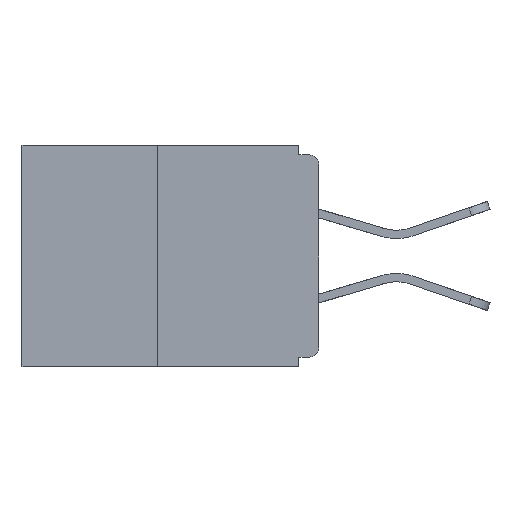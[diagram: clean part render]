
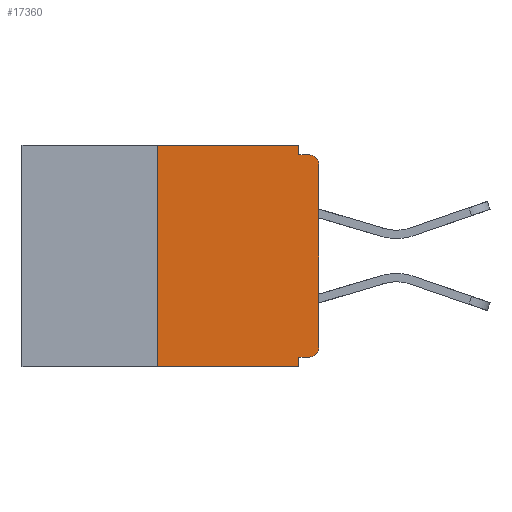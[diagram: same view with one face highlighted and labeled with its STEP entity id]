
A CAD part, left-side view. The second image highlights one B-rep face of the part: STEP entity #17360.
In plain terms, the highlighted planar face has unit normal (-1, 0, 0).
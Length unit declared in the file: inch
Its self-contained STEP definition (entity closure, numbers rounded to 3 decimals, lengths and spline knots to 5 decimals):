
#166 = ORIENTED_EDGE ( 'NONE', *, *, #1238, .T. ) ;
#215 = CARTESIAN_POINT ( 'NONE',  ( 0., 0., -0.328 ) ) ;
#246 = ORIENTED_EDGE ( 'NONE', *, *, #18057, .T. ) ;
#530 = VECTOR ( 'NONE', #8843, 39.37008 ) ;
#594 = DIRECTION ( 'NONE',  ( 0., 0., -1. ) ) ;
#1238 = EDGE_CURVE ( 'NONE', #21422, #5049, #30726, .T. ) ;
#1632 = VERTEX_POINT ( 'NONE', #28613 ) ;
#2028 = CARTESIAN_POINT ( 'NONE',  ( 0., 0., -0.313 ) ) ;
#2409 = ORIENTED_EDGE ( 'NONE', *, *, #9950, .F. ) ;
#2642 = AXIS2_PLACEMENT_3D ( 'NONE', #22882, #27794, #13150 ) ;
#2669 = CARTESIAN_POINT ( 'NONE',  ( 0., 0.015, -0.03 ) ) ;
#3594 = AXIS2_PLACEMENT_3D ( 'NONE', #27249, #15269, #594 ) ;
#4149 = VERTEX_POINT ( 'NONE', #10280 ) ;
#4864 = VERTEX_POINT ( 'NONE', #16593 ) ;
#5049 = VERTEX_POINT ( 'NONE', #30414 ) ;
#5520 = LINE ( 'NONE', #11395, #530 ) ;
#6552 = CARTESIAN_POINT ( 'NONE',  ( 0., 0.25, -0.343 ) ) ;
#7252 = EDGE_CURVE ( 'NONE', #4864, #5049, #5520, .T. ) ;
#7854 = VERTEX_POINT ( 'NONE', #2028 ) ;
#7888 = DIRECTION ( 'NONE',  ( 0., 0., -1. ) ) ;
#8566 = ORIENTED_EDGE ( 'NONE', *, *, #23306, .F. ) ;
#8618 = VECTOR ( 'NONE', #13808, 39.37008 ) ;
#8843 = DIRECTION ( 'NONE',  ( 0., 0., -1. ) ) ;
#9936 = VERTEX_POINT ( 'NONE', #29836 ) ;
#9950 = EDGE_CURVE ( 'NONE', #28685, #4864, #17190, .T. ) ;
#10280 = CARTESIAN_POINT ( 'NONE',  ( 0., 0.031, 0. ) ) ;
#10891 = DIRECTION ( 'NONE',  ( 0., -1., 0. ) ) ;
#10930 = LINE ( 'NONE', #18303, #8618 ) ;
#11076 = ORIENTED_EDGE ( 'NONE', *, *, #7252, .F. ) ;
#11395 = CARTESIAN_POINT ( 'NONE',  ( 0., 0.031, -0.343 ) ) ;
#11702 = VECTOR ( 'NONE', #31525, 39.37008 ) ;
#12018 = FACE_OUTER_BOUND ( 'NONE', #13596, .T. ) ;
#12447 = EDGE_CURVE ( 'NONE', #7854, #9936, #10930, .T. ) ;
#12721 = CARTESIAN_POINT ( 'NONE',  ( 0., 0.031, 0. ) ) ;
#13150 = DIRECTION ( 'NONE',  ( 0., 0., -1. ) ) ;
#13263 = CARTESIAN_POINT ( 'NONE',  ( 0., 0., -0.015 ) ) ;
#13403 = VECTOR ( 'NONE', #15731, 39.37008 ) ;
#13472 = EDGE_CURVE ( 'NONE', #1632, #30831, #26782, .T. ) ;
#13555 = ORIENTED_EDGE ( 'NONE', *, *, #15837, .F. ) ;
#13568 = CARTESIAN_POINT ( 'NONE',  ( 0., 0.46, 0. ) ) ;
#13596 = EDGE_LOOP ( 'NONE', ( #8566, #13555, #166, #11076, #2409, #246, #28429, #24397, #29983, #27112 ) ) ;
#13808 = DIRECTION ( 'NONE',  ( 0., 0., 1. ) ) ;
#14396 = EDGE_CURVE ( 'NONE', #9936, #30831, #28247, .T. ) ;
#14559 = CARTESIAN_POINT ( 'NONE',  ( 0., 0.25, 0. ) ) ;
#14901 = DIRECTION ( 'NONE',  ( 0., 1., 0. ) ) ;
#15269 = DIRECTION ( 'NONE',  ( -1., 0., 0. ) ) ;
#15716 = PLANE ( 'NONE',  #2642 ) ;
#15731 = DIRECTION ( 'NONE',  ( 0., -1., 0. ) ) ;
#15837 = EDGE_CURVE ( 'NONE', #21422, #19242, #24369, .T. ) ;
#16593 = CARTESIAN_POINT ( 'NONE',  ( 0., 0.031, -0.328 ) ) ;
#16851 = LINE ( 'NONE', #13568, #21045 ) ;
#17190 = LINE ( 'NONE', #215, #27528 ) ;
#17360 = ADVANCED_FACE ( 'NONE', ( #12018 ), #15716, .F. ) ;
#18057 = EDGE_CURVE ( 'NONE', #28685, #7854, #22308, .T. ) ;
#18303 = CARTESIAN_POINT ( 'NONE',  ( 0., 0., 0. ) ) ;
#19242 = VERTEX_POINT ( 'NONE', #27260 ) ;
#19511 = VECTOR ( 'NONE', #29917, 39.37008 ) ;
#21045 = VECTOR ( 'NONE', #10891, 39.37008 ) ;
#21422 = VERTEX_POINT ( 'NONE', #6552 ) ;
#22308 = CIRCLE ( 'NONE', #3594, 0.015 ) ;
#22882 = CARTESIAN_POINT ( 'NONE',  ( 0., 0.46, 0. ) ) ;
#23306 = EDGE_CURVE ( 'NONE', #19242, #4149, #16851, .T. ) ;
#24369 = LINE ( 'NONE', #14559, #11702 ) ;
#24397 = ORIENTED_EDGE ( 'NONE', *, *, #14396, .T. ) ;
#24817 = DIRECTION ( 'NONE',  ( 0., -1., 0. ) ) ;
#26782 = LINE ( 'NONE', #13263, #13403 ) ;
#27112 = ORIENTED_EDGE ( 'NONE', *, *, #30425, .F. ) ;
#27249 = CARTESIAN_POINT ( 'NONE',  ( 0., 0.015, -0.313 ) ) ;
#27260 = CARTESIAN_POINT ( 'NONE',  ( 0., 0.25, 0. ) ) ;
#27528 = VECTOR ( 'NONE', #14901, 39.37008 ) ;
#27687 = VECTOR ( 'NONE', #24817, 39.37008 ) ;
#27794 = DIRECTION ( 'NONE',  ( 1., 0., 0. ) ) ;
#28247 = CIRCLE ( 'NONE', #31152, 0.015 ) ;
#28300 = LINE ( 'NONE', #12721, #19511 ) ;
#28429 = ORIENTED_EDGE ( 'NONE', *, *, #12447, .T. ) ;
#28613 = CARTESIAN_POINT ( 'NONE',  ( 0., 0.031, -0.015 ) ) ;
#28685 = VERTEX_POINT ( 'NONE', #29786 ) ;
#29600 = CARTESIAN_POINT ( 'NONE',  ( 0., 0.46, -0.343 ) ) ;
#29786 = CARTESIAN_POINT ( 'NONE',  ( 0., 0.015, -0.328 ) ) ;
#29836 = CARTESIAN_POINT ( 'NONE',  ( 0., 0., -0.03 ) ) ;
#29907 = DIRECTION ( 'NONE',  ( -1., 0., 0. ) ) ;
#29917 = DIRECTION ( 'NONE',  ( 0., 0., -1. ) ) ;
#29983 = ORIENTED_EDGE ( 'NONE', *, *, #13472, .F. ) ;
#30414 = CARTESIAN_POINT ( 'NONE',  ( 0., 0.031, -0.343 ) ) ;
#30425 = EDGE_CURVE ( 'NONE', #4149, #1632, #28300, .T. ) ;
#30698 = CARTESIAN_POINT ( 'NONE',  ( 0., 0.015, -0.015 ) ) ;
#30726 = LINE ( 'NONE', #29600, #27687 ) ;
#30831 = VERTEX_POINT ( 'NONE', #30698 ) ;
#31152 = AXIS2_PLACEMENT_3D ( 'NONE', #2669, #29907, #7888 ) ;
#31525 = DIRECTION ( 'NONE',  ( 0., 0., 1. ) ) ;
